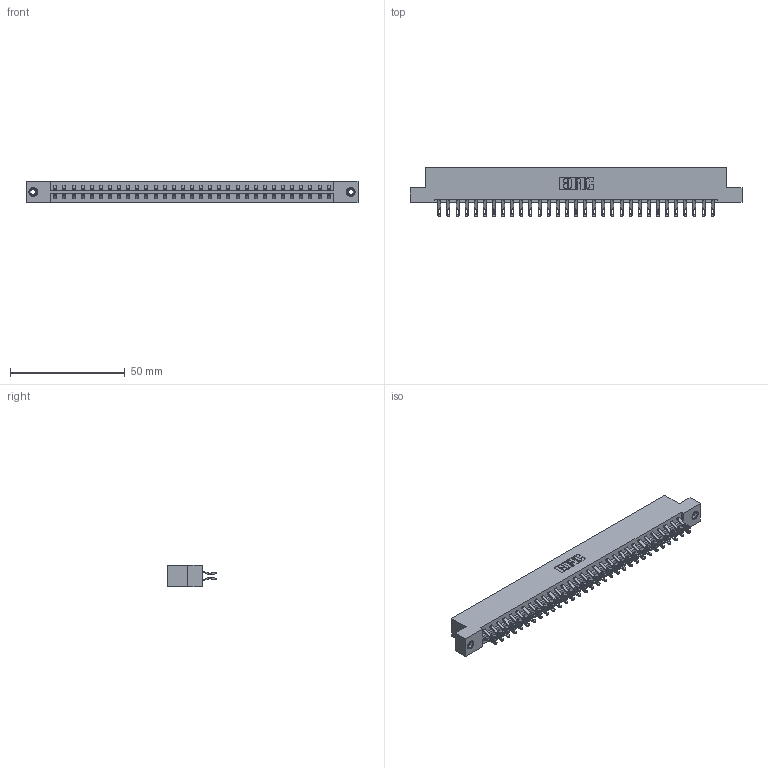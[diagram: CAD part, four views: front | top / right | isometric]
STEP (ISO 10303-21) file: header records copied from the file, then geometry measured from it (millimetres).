
FILE_DESCRIPTION (( 'STEP AP203' ), '1' );
FILE_NAME ('333-062-555-208.STEP', '2018-08-04T08:52:21', ( '' ), ( '' ), 'SwSTEP 2.0', 'SolidWorks 2016', '' );
FILE_SCHEMA (( 'CONFIG_CONTROL_DESIGN' ));
Length unit declared in the file: inch
Products named in the file (4): 333 Part_Flush - .156 Dia - TI; 345-292-001_555 Tail; 345-250-001_345-250-003-102; 333-062-555-208
Assembly tree (65 placements, depth 2):
  333-062-555-208
    333 Part_Flush - .156 Dia - TI
    345-292-001_555 Tail  x62
    345-250-001_345-250-003-102  x2
Bounding box: 144.37 x 21.47 x 9.4 mm (x, y, z)
Volume: 14810.2 mm3; surface area: 18085.4 mm2
Topology: 65 solids, 65 shells, 3770 faces, 11793 edges, 7854 vertices
Faces by surface type: plane 2210, cylinder 1544, cone 12, torus 4
Entity records: 22878 total; most frequent: CARTESIAN_POINT 3823, ORIENTED_EDGE 3722, DIRECTION 3287, EDGE_CURVE 1861, LINE 1693, VECTOR 1693, VERTEX_POINT 1236, AXIS2_PLACEMENT_3D 797
